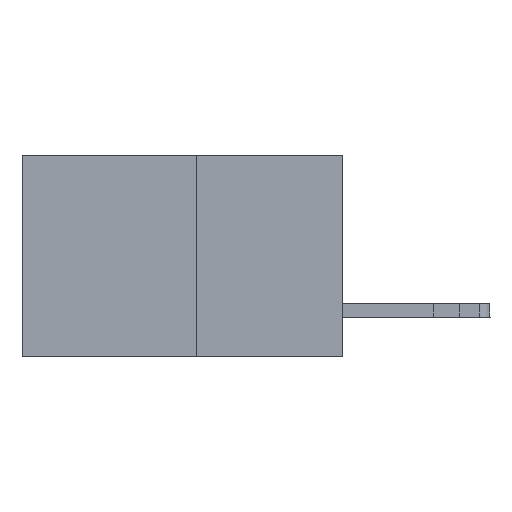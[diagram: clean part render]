
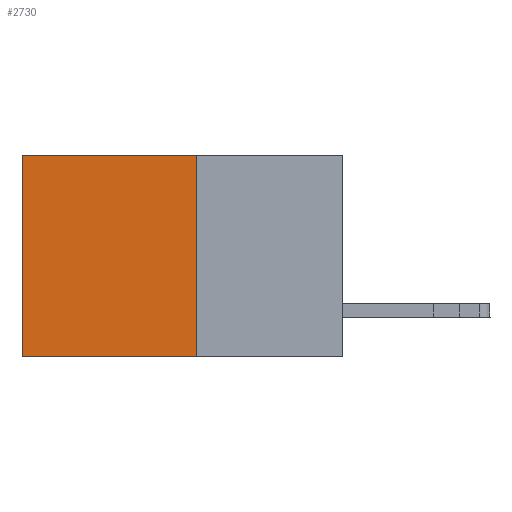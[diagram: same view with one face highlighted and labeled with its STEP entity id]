
A CAD part, left-side view. The second image highlights one B-rep face of the part: STEP entity #2730.
In plain terms, the highlighted planar face has unit normal (-1, 0, 0).
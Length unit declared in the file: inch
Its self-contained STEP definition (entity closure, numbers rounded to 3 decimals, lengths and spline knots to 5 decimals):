
#1218 = LINE ( 'NONE', #11258, #23401 ) ;
#1587 = VERTEX_POINT ( 'NONE', #23449 ) ;
#2655 = EDGE_CURVE ( 'NONE', #1587, #15298, #1218, .T. ) ;
#2730 = ADVANCED_FACE ( 'NONE', ( #5872 ), #22990, .F. ) ;
#3854 = DIRECTION ( 'NONE',  ( 1., 0., 0. ) ) ;
#5816 = LINE ( 'NONE', #24498, #29406 ) ;
#5872 = FACE_OUTER_BOUND ( 'NONE', #24263, .T. ) ;
#9329 = CARTESIAN_POINT ( 'NONE',  ( 0.277, 0.27, -0.37 ) ) ;
#10286 = ORIENTED_EDGE ( 'NONE', *, *, #24136, .F. ) ;
#10640 = CARTESIAN_POINT ( 'NONE',  ( 0.277, 0.27, -0.37 ) ) ;
#10753 = DIRECTION ( 'NONE',  ( 0., 0., -1. ) ) ;
#11258 = CARTESIAN_POINT ( 'NONE',  ( 0.277, 0.27, -0.37 ) ) ;
#11379 = VERTEX_POINT ( 'NONE', #25016 ) ;
#12110 = CARTESIAN_POINT ( 'NONE',  ( 0.277, 0.27, 0. ) ) ;
#12894 = ORIENTED_EDGE ( 'NONE', *, *, #2655, .F. ) ;
#13415 = DIRECTION ( 'NONE',  ( 0., 0., -1. ) ) ;
#13943 = ORIENTED_EDGE ( 'NONE', *, *, #20056, .T. ) ;
#15298 = VERTEX_POINT ( 'NONE', #9329 ) ;
#15301 = LINE ( 'NONE', #10640, #20463 ) ;
#15448 = CARTESIAN_POINT ( 'NONE',  ( 0.277, 0.27, -0.37 ) ) ;
#17927 = DIRECTION ( 'NONE',  ( 0., 0., -1. ) ) ;
#19244 = DIRECTION ( 'NONE',  ( 0., 1., 0. ) ) ;
#19546 = VERTEX_POINT ( 'NONE', #23422 ) ;
#19786 = EDGE_CURVE ( 'NONE', #19546, #11379, #5816, .T. ) ;
#20056 = EDGE_CURVE ( 'NONE', #1587, #19546, #28183, .T. ) ;
#20463 = VECTOR ( 'NONE', #24691, 39.37008 ) ;
#21981 = VECTOR ( 'NONE', #19244, 39.37008 ) ;
#22990 = PLANE ( 'NONE',  #25812 ) ;
#23401 = VECTOR ( 'NONE', #17927, 39.37008 ) ;
#23422 = CARTESIAN_POINT ( 'NONE',  ( 0.277, 0.59, 0. ) ) ;
#23449 = CARTESIAN_POINT ( 'NONE',  ( 0.277, 0.27, 0. ) ) ;
#24136 = EDGE_CURVE ( 'NONE', #15298, #11379, #15301, .T. ) ;
#24263 = EDGE_LOOP ( 'NONE', ( #26751, #10286, #12894, #13943 ) ) ;
#24498 = CARTESIAN_POINT ( 'NONE',  ( 0.277, 0.59, -0.37 ) ) ;
#24691 = DIRECTION ( 'NONE',  ( 0., 1., 0. ) ) ;
#25016 = CARTESIAN_POINT ( 'NONE',  ( 0.277, 0.59, -0.37 ) ) ;
#25812 = AXIS2_PLACEMENT_3D ( 'NONE', #15448, #3854, #13415 ) ;
#26751 = ORIENTED_EDGE ( 'NONE', *, *, #19786, .T. ) ;
#28183 = LINE ( 'NONE', #12110, #21981 ) ;
#29406 = VECTOR ( 'NONE', #10753, 39.37008 ) ;
